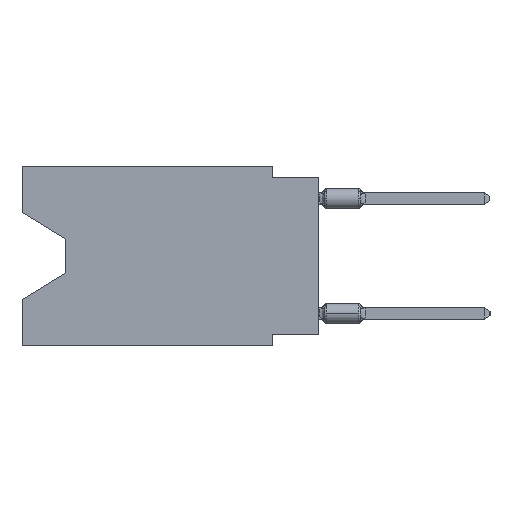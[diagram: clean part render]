
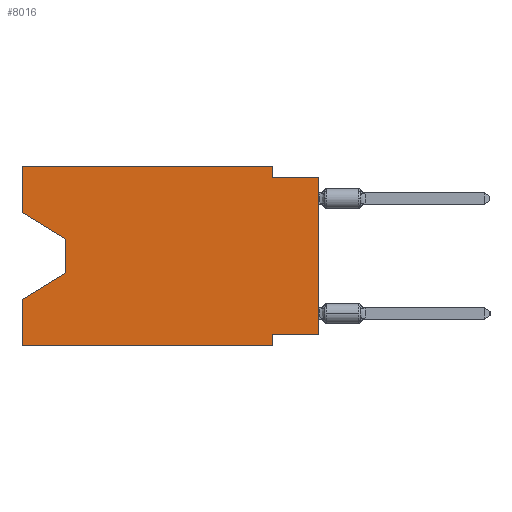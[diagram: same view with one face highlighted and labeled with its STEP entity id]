
A CAD part, left-side view. The second image highlights one B-rep face of the part: STEP entity #8016.
In plain terms, the highlighted planar face has unit normal (-1, 0, 0).
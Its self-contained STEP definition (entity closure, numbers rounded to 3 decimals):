
#359 = CARTESIAN_POINT ( 'NONE',  ( 0., 0., -9.271 ) ) ;
#1372 = EDGE_CURVE ( 'NONE', #26381, #20013, #6550, .T. ) ;
#2179 = CARTESIAN_POINT ( 'NONE',  ( 0., 2.54, -9.271 ) ) ;
#2364 = EDGE_CURVE ( 'NONE', #8634, #35840, #32065, .T. ) ;
#2396 = DIRECTION ( 'NONE',  ( 0., -0.855, -0.519 ) ) ;
#3136 = DIRECTION ( 'NONE',  ( 0., 1., 0. ) ) ;
#3737 = DIRECTION ( 'NONE',  ( 0., 0., -1. ) ) ;
#3997 = DIRECTION ( 'NONE',  ( 0., -1., 0. ) ) ;
#4658 = DIRECTION ( 'NONE',  ( 0., -1., 0. ) ) ;
#5162 = ORIENTED_EDGE ( 'NONE', *, *, #33607, .T. ) ;
#5210 = LINE ( 'NONE', #33693, #26853 ) ;
#5840 = CARTESIAN_POINT ( 'NONE',  ( 0., 2.54, 0. ) ) ;
#6550 = LINE ( 'NONE', #21043, #35979 ) ;
#6591 = CARTESIAN_POINT ( 'NONE',  ( 0., 0., -0.635 ) ) ;
#6630 = CARTESIAN_POINT ( 'NONE',  ( 0., 16.383, -9.906 ) ) ;
#6795 = VECTOR ( 'NONE', #3997, 1000. ) ;
#6957 = DIRECTION ( 'NONE',  ( 1., 0., 0. ) ) ;
#8016 = ADVANCED_FACE ( 'NONE', ( #31174 ), #9388, .F. ) ;
#8634 = VERTEX_POINT ( 'NONE', #2179 ) ;
#9267 = CARTESIAN_POINT ( 'NONE',  ( 0., 16.383, -2.546 ) ) ;
#9388 = PLANE ( 'NONE',  #34496 ) ;
#9747 = CARTESIAN_POINT ( 'NONE',  ( 0., 16.383, -7.36 ) ) ;
#10290 = EDGE_CURVE ( 'NONE', #27350, #21935, #28863, .T. ) ;
#10386 = VECTOR ( 'NONE', #13059, 1000. ) ;
#10390 = ORIENTED_EDGE ( 'NONE', *, *, #2364, .F. ) ;
#12188 = LINE ( 'NONE', #14799, #25385 ) ;
#12355 = DIRECTION ( 'NONE',  ( 0., 0., -1. ) ) ;
#12828 = VECTOR ( 'NONE', #33387, 1000. ) ;
#13059 = DIRECTION ( 'NONE',  ( 0., 0.855, -0.519 ) ) ;
#13264 = VECTOR ( 'NONE', #4658, 1000. ) ;
#13612 = EDGE_CURVE ( 'NONE', #13722, #19685, #34205, .T. ) ;
#13722 = VERTEX_POINT ( 'NONE', #6630 ) ;
#14799 = CARTESIAN_POINT ( 'NONE',  ( 0., 0., -0.635 ) ) ;
#15280 = ORIENTED_EDGE ( 'NONE', *, *, #32309, .F. ) ;
#15283 = CARTESIAN_POINT ( 'NONE',  ( 0., 16.383, 0. ) ) ;
#15290 = DIRECTION ( 'NONE',  ( 0., 0., -1. ) ) ;
#15889 = LINE ( 'NONE', #27243, #12828 ) ;
#16385 = VECTOR ( 'NONE', #31671, 1000. ) ;
#16575 = ORIENTED_EDGE ( 'NONE', *, *, #13612, .F. ) ;
#16857 = ORIENTED_EDGE ( 'NONE', *, *, #28486, .T. ) ;
#16878 = CARTESIAN_POINT ( 'NONE',  ( 0., 16.383, 0. ) ) ;
#17237 = CARTESIAN_POINT ( 'NONE',  ( 0., 13.97, -5.893 ) ) ;
#17744 = ORIENTED_EDGE ( 'NONE', *, *, #10290, .F. ) ;
#18010 = LINE ( 'NONE', #359, #19197 ) ;
#18323 = EDGE_CURVE ( 'NONE', #13722, #35840, #32965, .T. ) ;
#19000 = CARTESIAN_POINT ( 'NONE',  ( 0., 13.97, -5.893 ) ) ;
#19197 = VECTOR ( 'NONE', #3136, 1000. ) ;
#19685 = VERTEX_POINT ( 'NONE', #9747 ) ;
#20013 = VERTEX_POINT ( 'NONE', #29187 ) ;
#20036 = EDGE_CURVE ( 'NONE', #31774, #8634, #18010, .T. ) ;
#20391 = VERTEX_POINT ( 'NONE', #17237 ) ;
#20608 = CARTESIAN_POINT ( 'NONE',  ( 0., 2.54, -9.906 ) ) ;
#20733 = LINE ( 'NONE', #32117, #6795 ) ;
#21043 = CARTESIAN_POINT ( 'NONE',  ( 0., 2.54, 0. ) ) ;
#21758 = CARTESIAN_POINT ( 'NONE',  ( 0., 16.383, -9.906 ) ) ;
#21935 = VERTEX_POINT ( 'NONE', #15283 ) ;
#22054 = ORIENTED_EDGE ( 'NONE', *, *, #31550, .T. ) ;
#23193 = DIRECTION ( 'NONE',  ( 0., 0., 1. ) ) ;
#25376 = ORIENTED_EDGE ( 'NONE', *, *, #32852, .T. ) ;
#25385 = VECTOR ( 'NONE', #34928, 1000. ) ;
#25561 = CARTESIAN_POINT ( 'NONE',  ( 0., 16.383, 0. ) ) ;
#26023 = CARTESIAN_POINT ( 'NONE',  ( 0., 0., -9.271 ) ) ;
#26381 = VERTEX_POINT ( 'NONE', #5840 ) ;
#26396 = EDGE_LOOP ( 'NONE', ( #16857, #22054, #25376, #16575, #36375, #10390, #28835, #5162, #33552, #29065, #15280, #17744 ) ) ;
#26853 = VECTOR ( 'NONE', #2396, 1000. ) ;
#27243 = CARTESIAN_POINT ( 'NONE',  ( 0., 0., 0. ) ) ;
#27350 = VERTEX_POINT ( 'NONE', #9267 ) ;
#28486 = EDGE_CURVE ( 'NONE', #27350, #32193, #5210, .T. ) ;
#28835 = ORIENTED_EDGE ( 'NONE', *, *, #20036, .F. ) ;
#28863 = LINE ( 'NONE', #31857, #16385 ) ;
#29065 = ORIENTED_EDGE ( 'NONE', *, *, #1372, .F. ) ;
#29187 = CARTESIAN_POINT ( 'NONE',  ( 0., 2.54, -0.635 ) ) ;
#29246 = CARTESIAN_POINT ( 'NONE',  ( 0., 2.54, -9.906 ) ) ;
#29344 = VERTEX_POINT ( 'NONE', #6591 ) ;
#31174 = FACE_OUTER_BOUND ( 'NONE', #26396, .T. ) ;
#31306 = VECTOR ( 'NONE', #3737, 1000. ) ;
#31550 = EDGE_CURVE ( 'NONE', #32193, #20391, #35923, .T. ) ;
#31671 = DIRECTION ( 'NONE',  ( 0., 0., 1. ) ) ;
#31774 = VERTEX_POINT ( 'NONE', #26023 ) ;
#31857 = CARTESIAN_POINT ( 'NONE',  ( 0., 16.383, 0. ) ) ;
#32065 = LINE ( 'NONE', #29246, #31306 ) ;
#32117 = CARTESIAN_POINT ( 'NONE',  ( 0., 16.383, 0. ) ) ;
#32193 = VERTEX_POINT ( 'NONE', #33823 ) ;
#32309 = EDGE_CURVE ( 'NONE', #21935, #26381, #20733, .T. ) ;
#32852 = EDGE_CURVE ( 'NONE', #20391, #19685, #35618, .T. ) ;
#32950 = DIRECTION ( 'NONE',  ( 0., 0., -1. ) ) ;
#32965 = LINE ( 'NONE', #21758, #13264 ) ;
#33135 = CARTESIAN_POINT ( 'NONE',  ( 0., 13.97, -4.013 ) ) ;
#33387 = DIRECTION ( 'NONE',  ( 0., 0., 1. ) ) ;
#33552 = ORIENTED_EDGE ( 'NONE', *, *, #36293, .F. ) ;
#33607 = EDGE_CURVE ( 'NONE', #31774, #29344, #15889, .T. ) ;
#33693 = CARTESIAN_POINT ( 'NONE',  ( 0., 16.383, -2.546 ) ) ;
#33823 = CARTESIAN_POINT ( 'NONE',  ( 0., 13.97, -4.013 ) ) ;
#34205 = LINE ( 'NONE', #16878, #36046 ) ;
#34496 = AXIS2_PLACEMENT_3D ( 'NONE', #25561, #6957, #12355 ) ;
#34928 = DIRECTION ( 'NONE',  ( 0., -1., 0. ) ) ;
#35329 = VECTOR ( 'NONE', #32950, 1000. ) ;
#35618 = LINE ( 'NONE', #19000, #10386 ) ;
#35840 = VERTEX_POINT ( 'NONE', #20608 ) ;
#35923 = LINE ( 'NONE', #33135, #35329 ) ;
#35979 = VECTOR ( 'NONE', #15290, 1000. ) ;
#36046 = VECTOR ( 'NONE', #23193, 1000. ) ;
#36293 = EDGE_CURVE ( 'NONE', #20013, #29344, #12188, .T. ) ;
#36375 = ORIENTED_EDGE ( 'NONE', *, *, #18323, .T. ) ;
